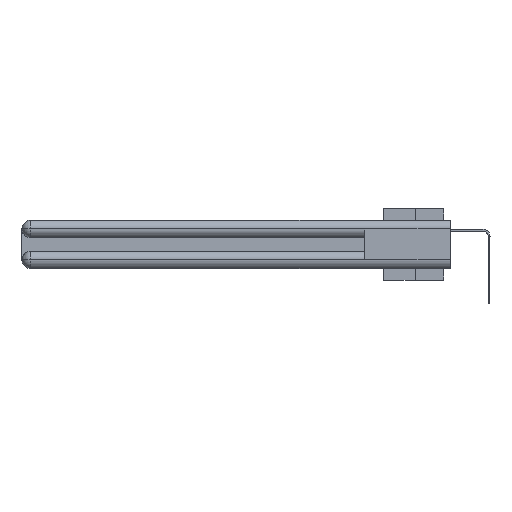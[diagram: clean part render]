
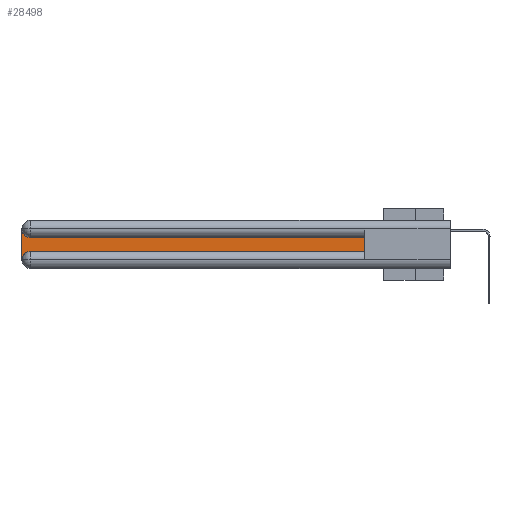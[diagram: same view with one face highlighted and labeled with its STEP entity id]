
A CAD part, left-side view. The second image highlights one B-rep face of the part: STEP entity #28498.
In plain terms, the highlighted planar face has unit normal (-1, 0, 0).
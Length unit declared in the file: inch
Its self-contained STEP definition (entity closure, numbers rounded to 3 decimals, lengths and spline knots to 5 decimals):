
#890 = ORIENTED_EDGE ( 'NONE', *, *, #19393, .T. ) ;
#1274 = EDGE_CURVE ( 'NONE', #1501, #23619, #27715, .T. ) ;
#1448 = ORIENTED_EDGE ( 'NONE', *, *, #23739, .T. ) ;
#1501 = VERTEX_POINT ( 'NONE', #23909 ) ;
#3864 = FACE_OUTER_BOUND ( 'NONE', #28316, .T. ) ;
#4303 = EDGE_CURVE ( 'NONE', #27935, #15325, #22850, .T. ) ;
#4817 = CARTESIAN_POINT ( 'NONE',  ( 0.075, 3., -0.2175 ) ) ;
#4880 = CARTESIAN_POINT ( 'NONE',  ( 0.075, 2.94, -0.1225 ) ) ;
#5675 = CARTESIAN_POINT ( 'NONE',  ( 0.075, 3., -0.0625 ) ) ;
#6546 = CARTESIAN_POINT ( 'NONE',  ( 0.075, 2.94, -0.2775 ) ) ;
#6706 = VECTOR ( 'NONE', #17884, 39.37008 ) ;
#7119 = VECTOR ( 'NONE', #27530, 39.37008 ) ;
#7130 = ORIENTED_EDGE ( 'NONE', *, *, #23402, .T. ) ;
#7235 = CARTESIAN_POINT ( 'NONE',  ( 0.075, 0.6, -0.2175 ) ) ;
#7300 = EDGE_CURVE ( 'NONE', #15325, #24035, #13986, .T. ) ;
#8528 = PLANE ( 'NONE',  #26978 ) ;
#9105 = DIRECTION ( 'NONE',  ( 0., 0., -1. ) ) ;
#9524 = ORIENTED_EDGE ( 'NONE', *, *, #7300, .T. ) ;
#9694 = ORIENTED_EDGE ( 'NONE', *, *, #4303, .T. ) ;
#10026 = LINE ( 'NONE', #13975, #7119 ) ;
#10297 = CARTESIAN_POINT ( 'NONE',  ( 0.075, 2.94, -0.2175 ) ) ;
#10677 = DIRECTION ( 'NONE',  ( 0., 0., -1. ) ) ;
#10917 = DIRECTION ( 'NONE',  ( 1., 0., 0. ) ) ;
#10947 = CARTESIAN_POINT ( 'NONE',  ( 0.075, 0.6, -0.1225 ) ) ;
#13975 = CARTESIAN_POINT ( 'NONE',  ( 0.075, 0.6, -0.2175 ) ) ;
#13986 = LINE ( 'NONE', #10947, #6706 ) ;
#14217 = DIRECTION ( 'NONE',  ( 0., 0., 1. ) ) ;
#14465 = LINE ( 'NONE', #4817, #20621 ) ;
#15325 = VERTEX_POINT ( 'NONE', #21689 ) ;
#17403 = CARTESIAN_POINT ( 'NONE',  ( 0.075, 0.6, -0.2175 ) ) ;
#17884 = DIRECTION ( 'NONE',  ( 0., 1., 0. ) ) ;
#19393 = EDGE_CURVE ( 'NONE', #23619, #27935, #10026, .T. ) ;
#20388 = DIRECTION ( 'NONE',  ( 0., 0., -1. ) ) ;
#20621 = VECTOR ( 'NONE', #21211, 39.37008 ) ;
#20758 = ORIENTED_EDGE ( 'NONE', *, *, #1274, .T. ) ;
#21101 = VERTEX_POINT ( 'NONE', #5675 ) ;
#21211 = DIRECTION ( 'NONE',  ( 0., 0., -1. ) ) ;
#21392 = VECTOR ( 'NONE', #14217, 39.37008 ) ;
#21689 = CARTESIAN_POINT ( 'NONE',  ( 0.075, 0.6, -0.1225 ) ) ;
#21887 = AXIS2_PLACEMENT_3D ( 'NONE', #29695, #10917, #20388 ) ;
#22383 = DIRECTION ( 'NONE',  ( 1., 0., 0. ) ) ;
#22551 = DIRECTION ( 'NONE',  ( 1., 0., 0. ) ) ;
#22850 = LINE ( 'NONE', #7235, #21392 ) ;
#23402 = EDGE_CURVE ( 'NONE', #21101, #1501, #14465, .T. ) ;
#23619 = VERTEX_POINT ( 'NONE', #10297 ) ;
#23739 = EDGE_CURVE ( 'NONE', #24035, #21101, #24994, .T. ) ;
#23909 = CARTESIAN_POINT ( 'NONE',  ( 0.075, 3., -0.2775 ) ) ;
#24035 = VERTEX_POINT ( 'NONE', #4880 ) ;
#24994 = CIRCLE ( 'NONE', #21887, 0.06 ) ;
#26978 = AXIS2_PLACEMENT_3D ( 'NONE', #29165, #22383, #10677 ) ;
#27530 = DIRECTION ( 'NONE',  ( 0., -1., 0. ) ) ;
#27715 = CIRCLE ( 'NONE', #28540, 0.06 ) ;
#27935 = VERTEX_POINT ( 'NONE', #17403 ) ;
#28316 = EDGE_LOOP ( 'NONE', ( #9524, #1448, #7130, #20758, #890, #9694 ) ) ;
#28498 = ADVANCED_FACE ( 'NONE', ( #3864 ), #8528, .F. ) ;
#28540 = AXIS2_PLACEMENT_3D ( 'NONE', #6546, #22551, #9105 ) ;
#29165 = CARTESIAN_POINT ( 'NONE',  ( 0.075, 3., -0.1225 ) ) ;
#29695 = CARTESIAN_POINT ( 'NONE',  ( 0.075, 2.94, -0.0625 ) ) ;
